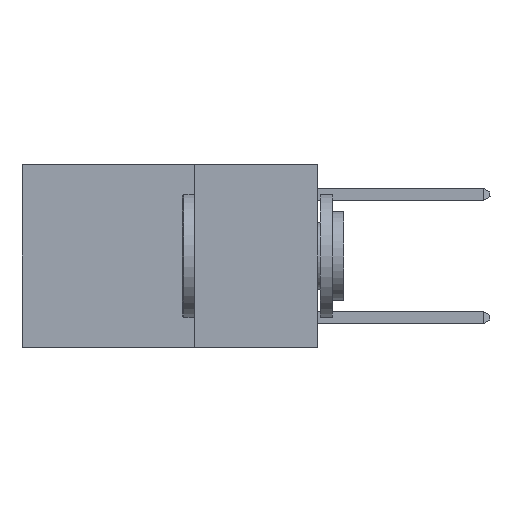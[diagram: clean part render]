
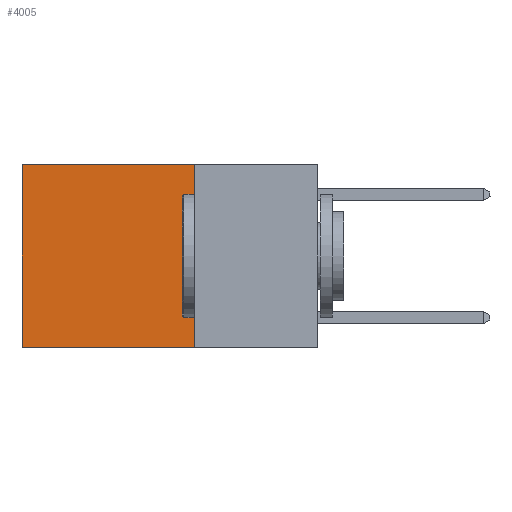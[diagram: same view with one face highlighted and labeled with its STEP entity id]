
A CAD part, left-side view. The second image highlights one B-rep face of the part: STEP entity #4005.
In plain terms, the highlighted planar face has unit normal (-1, 0, 0).
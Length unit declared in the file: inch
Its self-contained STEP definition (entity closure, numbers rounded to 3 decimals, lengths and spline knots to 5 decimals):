
#170 = CARTESIAN_POINT ( 'NONE',  ( 0.2625, 0.25, -0.37 ) ) ;
#407 = CARTESIAN_POINT ( 'NONE',  ( 0.2625, 0.25, 0. ) ) ;
#1652 = DIRECTION ( 'NONE',  ( 0., 1., 0. ) ) ;
#1954 = DIRECTION ( 'NONE',  ( 0., 0., -1. ) ) ;
#2519 = DIRECTION ( 'NONE',  ( 1., 0., 0. ) ) ;
#3288 = LINE ( 'NONE', #8733, #15868 ) ;
#4005 = ADVANCED_FACE ( 'NONE', ( #5107 ), #5194, .F. ) ;
#4075 = EDGE_LOOP ( 'NONE', ( #9897, #11083, #13794, #13867 ) ) ;
#4349 = VECTOR ( 'NONE', #9391, 39.37008 ) ;
#5107 = FACE_OUTER_BOUND ( 'NONE', #4075, .T. ) ;
#5194 = PLANE ( 'NONE',  #5981 ) ;
#5361 = CARTESIAN_POINT ( 'NONE',  ( 0.2625, 0.25, 0. ) ) ;
#5528 = EDGE_CURVE ( 'NONE', #12137, #7514, #3288, .T. ) ;
#5981 = AXIS2_PLACEMENT_3D ( 'NONE', #6711, #2519, #16379 ) ;
#6054 = LINE ( 'NONE', #407, #7594 ) ;
#6711 = CARTESIAN_POINT ( 'NONE',  ( 0.2625, 0.25, 0. ) ) ;
#7128 = VERTEX_POINT ( 'NONE', #5361 ) ;
#7187 = LINE ( 'NONE', #11140, #7934 ) ;
#7514 = VERTEX_POINT ( 'NONE', #14685 ) ;
#7594 = VECTOR ( 'NONE', #11435, 39.37008 ) ;
#7934 = VECTOR ( 'NONE', #1652, 39.37008 ) ;
#8416 = EDGE_CURVE ( 'NONE', #15467, #7514, #14999, .T. ) ;
#8733 = CARTESIAN_POINT ( 'NONE',  ( 0.2625, 0.6, 0. ) ) ;
#9034 = CARTESIAN_POINT ( 'NONE',  ( 0.2625, 0.6, 0. ) ) ;
#9391 = DIRECTION ( 'NONE',  ( 0., 1., 0. ) ) ;
#9897 = ORIENTED_EDGE ( 'NONE', *, *, #5528, .T. ) ;
#10506 = CARTESIAN_POINT ( 'NONE',  ( 0.2625, 0.25, -0.37 ) ) ;
#11083 = ORIENTED_EDGE ( 'NONE', *, *, #8416, .F. ) ;
#11140 = CARTESIAN_POINT ( 'NONE',  ( 0.2625, 0.25, 0. ) ) ;
#11435 = DIRECTION ( 'NONE',  ( 0., 0., -1. ) ) ;
#11539 = EDGE_CURVE ( 'NONE', #7128, #15467, #6054, .T. ) ;
#12137 = VERTEX_POINT ( 'NONE', #9034 ) ;
#13794 = ORIENTED_EDGE ( 'NONE', *, *, #11539, .F. ) ;
#13867 = ORIENTED_EDGE ( 'NONE', *, *, #15653, .T. ) ;
#14685 = CARTESIAN_POINT ( 'NONE',  ( 0.2625, 0.6, -0.37 ) ) ;
#14999 = LINE ( 'NONE', #170, #4349 ) ;
#15467 = VERTEX_POINT ( 'NONE', #10506 ) ;
#15653 = EDGE_CURVE ( 'NONE', #7128, #12137, #7187, .T. ) ;
#15868 = VECTOR ( 'NONE', #1954, 39.37008 ) ;
#16379 = DIRECTION ( 'NONE',  ( 0., 0., -1. ) ) ;
